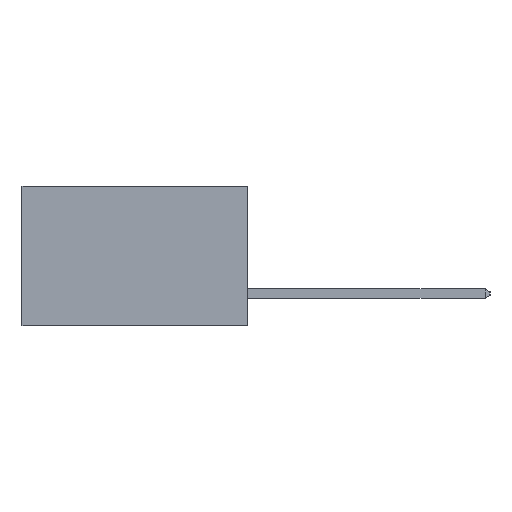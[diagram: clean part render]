
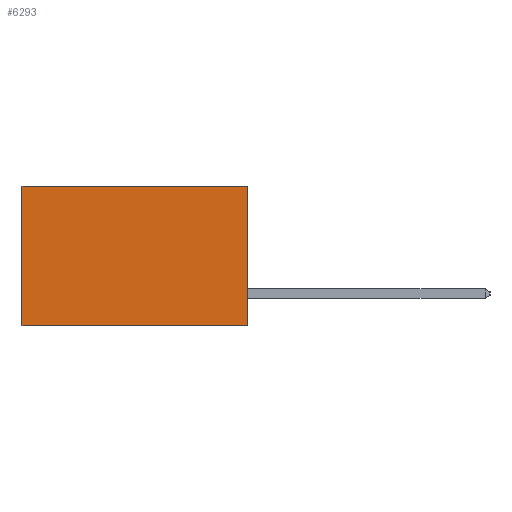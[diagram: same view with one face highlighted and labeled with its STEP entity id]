
A CAD part, left-side view. The second image highlights one B-rep face of the part: STEP entity #6293.
In plain terms, the highlighted planar face has unit normal (-1, 0, 0).
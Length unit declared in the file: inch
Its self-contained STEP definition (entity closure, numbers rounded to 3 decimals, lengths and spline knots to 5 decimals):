
#102 = CARTESIAN_POINT ( 'NONE',  ( 0.298, 0., 0. ) ) ;
#1137 = FACE_OUTER_BOUND ( 'NONE', #17107, .T. ) ;
#2147 = LINE ( 'NONE', #102, #22733 ) ;
#2454 = VERTEX_POINT ( 'NONE', #22720 ) ;
#4293 = AXIS2_PLACEMENT_3D ( 'NONE', #19284, #19363, #7114 ) ;
#4642 = VECTOR ( 'NONE', #19556, 39.37008 ) ;
#4968 = PLANE ( 'NONE',  #4293 ) ;
#5311 = LINE ( 'NONE', #7317, #4642 ) ;
#6210 = DIRECTION ( 'NONE',  ( 0., 1., 0. ) ) ;
#6293 = ADVANCED_FACE ( 'NONE', ( #1137 ), #4968, .F. ) ;
#6338 = DIRECTION ( 'NONE',  ( 0., 0., -1. ) ) ;
#6439 = CARTESIAN_POINT ( 'NONE',  ( 0.298, 0., 0. ) ) ;
#7114 = DIRECTION ( 'NONE',  ( 0., 0., -1. ) ) ;
#7317 = CARTESIAN_POINT ( 'NONE',  ( 0.298, 0., 0. ) ) ;
#8849 = ORIENTED_EDGE ( 'NONE', *, *, #25996, .F. ) ;
#9890 = CARTESIAN_POINT ( 'NONE',  ( 0.298, 0., -0.37 ) ) ;
#10532 = CARTESIAN_POINT ( 'NONE',  ( 0.298, 0.6, 0. ) ) ;
#10665 = LINE ( 'NONE', #10532, #21433 ) ;
#12704 = DIRECTION ( 'NONE',  ( 0., 1., 0. ) ) ;
#13839 = EDGE_CURVE ( 'NONE', #19779, #23384, #5311, .T. ) ;
#13949 = VECTOR ( 'NONE', #6210, 39.37008 ) ;
#15542 = ORIENTED_EDGE ( 'NONE', *, *, #13839, .F. ) ;
#16520 = CARTESIAN_POINT ( 'NONE',  ( 0.298, 0., -0.37 ) ) ;
#17107 = EDGE_LOOP ( 'NONE', ( #19993, #8849, #15542, #21753 ) ) ;
#17885 = CARTESIAN_POINT ( 'NONE',  ( 0.298, 0.6, -0.37 ) ) ;
#19283 = LINE ( 'NONE', #16520, #13949 ) ;
#19284 = CARTESIAN_POINT ( 'NONE',  ( 0.298, 0., 0. ) ) ;
#19363 = DIRECTION ( 'NONE',  ( 1., 0., 0. ) ) ;
#19556 = DIRECTION ( 'NONE',  ( 0., 0., -1. ) ) ;
#19779 = VERTEX_POINT ( 'NONE', #6439 ) ;
#19993 = ORIENTED_EDGE ( 'NONE', *, *, #25410, .T. ) ;
#21433 = VECTOR ( 'NONE', #6338, 39.37008 ) ;
#21753 = ORIENTED_EDGE ( 'NONE', *, *, #26406, .T. ) ;
#22720 = CARTESIAN_POINT ( 'NONE',  ( 0.298, 0.6, 0. ) ) ;
#22733 = VECTOR ( 'NONE', #12704, 39.37008 ) ;
#23384 = VERTEX_POINT ( 'NONE', #9890 ) ;
#24603 = VERTEX_POINT ( 'NONE', #17885 ) ;
#25410 = EDGE_CURVE ( 'NONE', #2454, #24603, #10665, .T. ) ;
#25996 = EDGE_CURVE ( 'NONE', #23384, #24603, #19283, .T. ) ;
#26406 = EDGE_CURVE ( 'NONE', #19779, #2454, #2147, .T. ) ;
